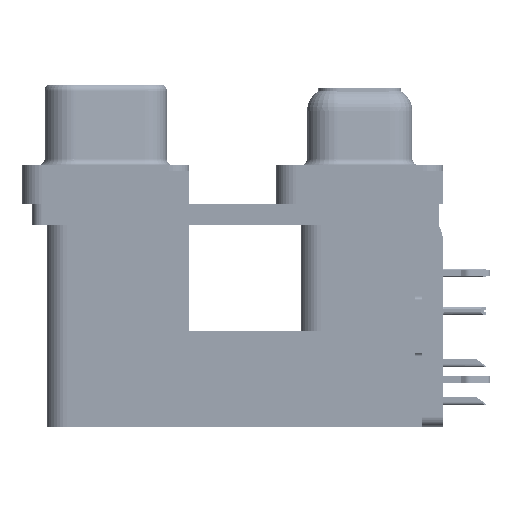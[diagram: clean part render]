
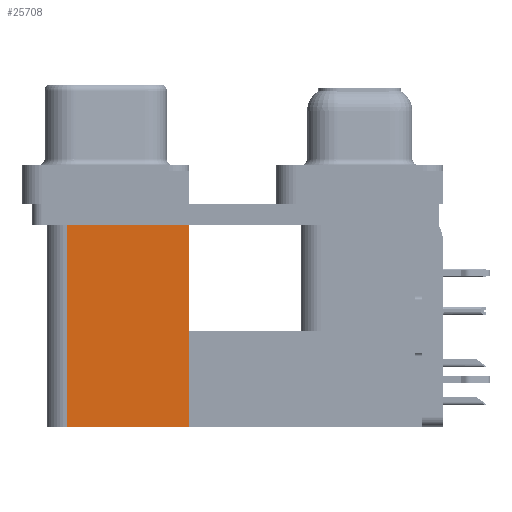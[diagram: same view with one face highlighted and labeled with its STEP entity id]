
A CAD part, left-side view. The second image highlights one B-rep face of the part: STEP entity #25708.
In plain terms, the highlighted planar face has unit normal (-1, 0, 0).
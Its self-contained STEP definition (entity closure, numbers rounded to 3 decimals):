
#1 = VECTOR ( 'NONE', #23085, 1000. ) ;
#2719 = LINE ( 'NONE', #40785, #8780 ) ;
#3189 = DIRECTION ( 'NONE',  ( 0., 1., 0. ) ) ;
#3803 = CARTESIAN_POINT ( 'NONE',  ( 3.79, 12.775, -19.2 ) ) ;
#7952 = ORIENTED_EDGE ( 'NONE', *, *, #16330, .T. ) ;
#8780 = VECTOR ( 'NONE', #41849, 1000. ) ;
#12097 = EDGE_LOOP ( 'NONE', ( #7952, #14273, #51379, #59124 ) ) ;
#13021 = AXIS2_PLACEMENT_3D ( 'NONE', #28789, #67212, #34462 ) ;
#14273 = ORIENTED_EDGE ( 'NONE', *, *, #18951, .F. ) ;
#14569 = LINE ( 'NONE', #19560, #18955 ) ;
#16330 = EDGE_CURVE ( 'NONE', #51541, #54257, #14569, .T. ) ;
#17709 = VECTOR ( 'NONE', #20646, 1000. ) ;
#18951 = EDGE_CURVE ( 'NONE', #20429, #54257, #2719, .T. ) ;
#18955 = VECTOR ( 'NONE', #3189, 1000. ) ;
#19560 = CARTESIAN_POINT ( 'NONE',  ( 3.79, 12.775, -2.5 ) ) ;
#20429 = VERTEX_POINT ( 'NONE', #63473 ) ;
#20646 = DIRECTION ( 'NONE',  ( 0., 0., 1. ) ) ;
#22743 = CARTESIAN_POINT ( 'NONE',  ( 3.79, 12.775, -19.2 ) ) ;
#23085 = DIRECTION ( 'NONE',  ( 0., 1., 0. ) ) ;
#25708 = ADVANCED_FACE ( 'NONE', ( #46550 ), #61509, .F. ) ;
#26340 = LINE ( 'NONE', #69409, #17709 ) ;
#27178 = EDGE_CURVE ( 'NONE', #60086, #51541, #26340, .T. ) ;
#28789 = CARTESIAN_POINT ( 'NONE',  ( 3.79, 12.775, -19.2 ) ) ;
#34462 = DIRECTION ( 'NONE',  ( 0., 1., 0. ) ) ;
#40785 = CARTESIAN_POINT ( 'NONE',  ( 3.79, 21.975, -19.2 ) ) ;
#41849 = DIRECTION ( 'NONE',  ( 0., 0., 1. ) ) ;
#46550 = FACE_OUTER_BOUND ( 'NONE', #12097, .T. ) ;
#47176 = EDGE_CURVE ( 'NONE', #60086, #20429, #65804, .T. ) ;
#48722 = CARTESIAN_POINT ( 'NONE',  ( 3.79, 21.975, -2.5 ) ) ;
#51379 = ORIENTED_EDGE ( 'NONE', *, *, #47176, .F. ) ;
#51541 = VERTEX_POINT ( 'NONE', #56553 ) ;
#54257 = VERTEX_POINT ( 'NONE', #48722 ) ;
#56553 = CARTESIAN_POINT ( 'NONE',  ( 3.79, 12.775, -2.5 ) ) ;
#59124 = ORIENTED_EDGE ( 'NONE', *, *, #27178, .T. ) ;
#60086 = VERTEX_POINT ( 'NONE', #3803 ) ;
#61509 = PLANE ( 'NONE',  #13021 ) ;
#63473 = CARTESIAN_POINT ( 'NONE',  ( 3.79, 21.975, -19.2 ) ) ;
#65804 = LINE ( 'NONE', #22743, #1 ) ;
#67212 = DIRECTION ( 'NONE',  ( 1., 0., 0. ) ) ;
#69409 = CARTESIAN_POINT ( 'NONE',  ( 3.79, 12.775, -19.2 ) ) ;
